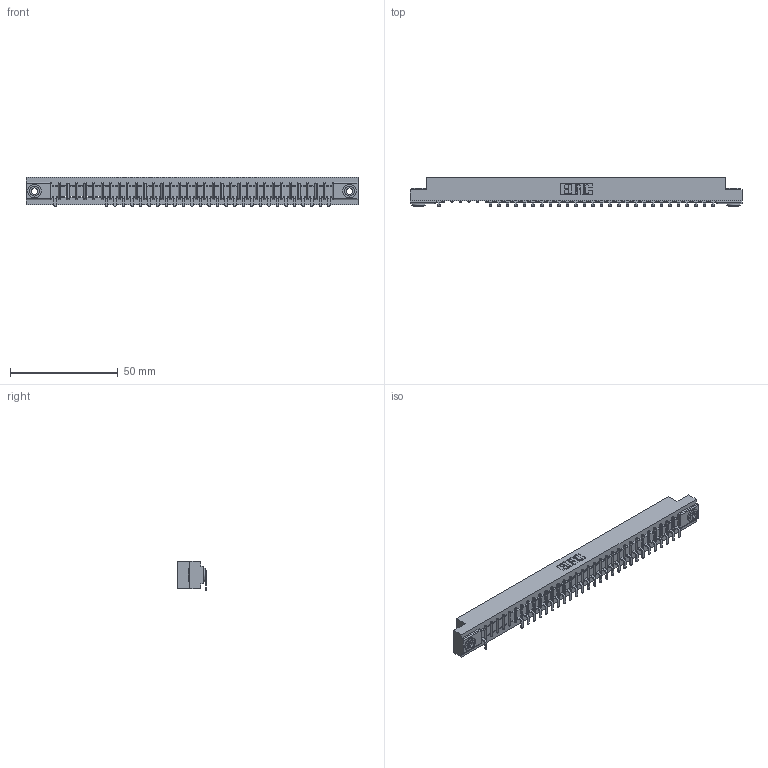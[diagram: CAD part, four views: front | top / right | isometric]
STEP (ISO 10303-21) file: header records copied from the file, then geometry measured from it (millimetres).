
FILE_DESCRIPTION (( 'STEP AP203' ), '1' );
FILE_NAME ('357-033-553-103.STEP', '2018-08-10T01:33:35', ( '' ), ( '' ), 'SwSTEP 2.0', 'SolidWorks 2016', '' );
FILE_SCHEMA (( 'CONFIG_CONTROL_DESIGN' ));
Length unit declared in the file: inch
Products named in the file (4): 307 Part_.156 Dia Mounting Holes; 307-290-002_553; 345-250-002_345-250-002-102; 357-033-553-103
Assembly tree (31 placements, depth 2):
  357-033-553-103
    307 Part_.156 Dia Mounting Holes
    307-290-002_553  x28
    345-250-002_345-250-002-102  x2
Bounding box: 153.77 x 13.36 x 13.5 mm (x, y, z)
Volume: 16244.9 mm3; surface area: 19546.5 mm2
Topology: 31 solids, 31 shells, 2488 faces, 7587 edges, 4962 vertices
Faces by surface type: plane 1470, cylinder 942, sphere 68, cone 8
Entity records: 31159 total; most frequent: CARTESIAN_POINT 5256, ORIENTED_EDGE 5242, DIRECTION 5121, EDGE_CURVE 2621, VECTOR 1995, LINE 1995, VERTEX_POINT 1698, AXIS2_PLACEMENT_3D 1563
